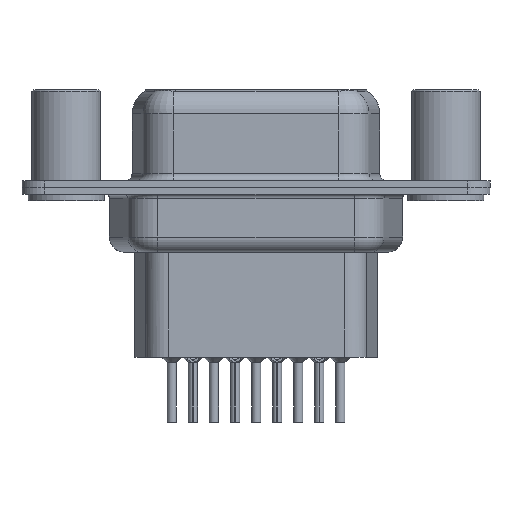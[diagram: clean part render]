
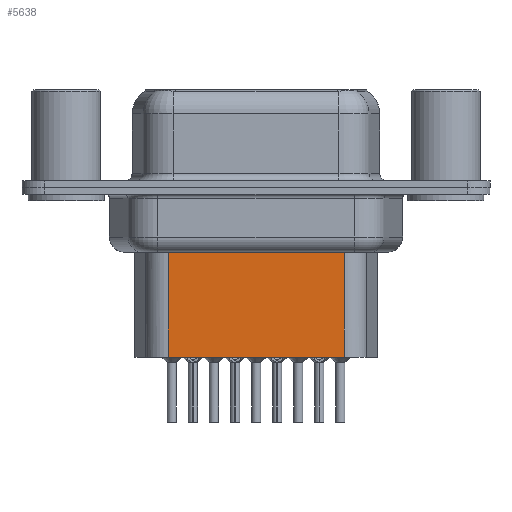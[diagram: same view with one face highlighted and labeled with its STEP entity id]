
A CAD part, front view. The second image highlights one B-rep face of the part: STEP entity #5638.
In plain terms, the highlighted planar face has unit normal (0, -1, 0).
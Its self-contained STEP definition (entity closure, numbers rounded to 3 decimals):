
#329 = ORIENTED_EDGE ( 'NONE', *, *, #17646, .F. ) ;
#628 = DIRECTION ( 'NONE',  ( 0., -1., 0. ) ) ;
#1397 = DIRECTION ( 'NONE',  ( -1., 0., 0. ) ) ;
#1409 = CARTESIAN_POINT ( 'NONE',  ( 18.294, -3.5, -3.1 ) ) ;
#1508 = ORIENTED_EDGE ( 'NONE', *, *, #8122, .T. ) ;
#1688 = ORIENTED_EDGE ( 'NONE', *, *, #22270, .F. ) ;
#2204 = FACE_OUTER_BOUND ( 'NONE', #20618, .T. ) ;
#2476 = VECTOR ( 'NONE', #3000, 1000. ) ;
#3000 = DIRECTION ( 'NONE',  ( 0., 0., -1. ) ) ;
#3358 = VERTEX_POINT ( 'NONE', #3954 ) ;
#3724 = CARTESIAN_POINT ( 'NONE',  ( 6.706, -3.5, -11.15 ) ) ;
#3954 = CARTESIAN_POINT ( 'NONE',  ( 18.294, -3.5, -11.15 ) ) ;
#4820 = VERTEX_POINT ( 'NONE', #20271 ) ;
#4893 = LINE ( 'NONE', #1409, #18375 ) ;
#5421 = VECTOR ( 'NONE', #14647, 1000. ) ;
#5638 = ADVANCED_FACE ( 'NONE', ( #2204 ), #5681, .T. ) ;
#5681 = PLANE ( 'NONE',  #8793 ) ;
#6378 = EDGE_CURVE ( 'NONE', #20563, #20127, #20225, .T. ) ;
#6590 = CARTESIAN_POINT ( 'NONE',  ( 6.706, -3.5, -3.1 ) ) ;
#7725 = LINE ( 'NONE', #16132, #5421 ) ;
#7826 = CARTESIAN_POINT ( 'NONE',  ( 6.459, -3.5, -4.097 ) ) ;
#8049 = LINE ( 'NONE', #7826, #21793 ) ;
#8122 = EDGE_CURVE ( 'NONE', #4820, #20563, #8049, .T. ) ;
#8793 = AXIS2_PLACEMENT_3D ( 'NONE', #9207, #628, #14430 ) ;
#9207 = CARTESIAN_POINT ( 'NONE',  ( 6.706, -3.5, -3.1 ) ) ;
#10901 = ORIENTED_EDGE ( 'NONE', *, *, #6378, .T. ) ;
#11977 = CARTESIAN_POINT ( 'NONE',  ( 6.706, -3.5, -4.097 ) ) ;
#13745 = DIRECTION ( 'NONE',  ( 0., 0., -1. ) ) ;
#14430 = DIRECTION ( 'NONE',  ( 1., 0., 0. ) ) ;
#14647 = DIRECTION ( 'NONE',  ( -1., 0., 0. ) ) ;
#16132 = CARTESIAN_POINT ( 'NONE',  ( 6.706, -3.5, -11.15 ) ) ;
#17646 = EDGE_CURVE ( 'NONE', #4820, #3358, #4893, .T. ) ;
#18375 = VECTOR ( 'NONE', #13745, 1000. ) ;
#20127 = VERTEX_POINT ( 'NONE', #3724 ) ;
#20225 = LINE ( 'NONE', #6590, #2476 ) ;
#20271 = CARTESIAN_POINT ( 'NONE',  ( 18.294, -3.5, -4.097 ) ) ;
#20563 = VERTEX_POINT ( 'NONE', #11977 ) ;
#20618 = EDGE_LOOP ( 'NONE', ( #329, #1508, #10901, #1688 ) ) ;
#21793 = VECTOR ( 'NONE', #1397, 1000. ) ;
#22270 = EDGE_CURVE ( 'NONE', #3358, #20127, #7725, .T. ) ;
